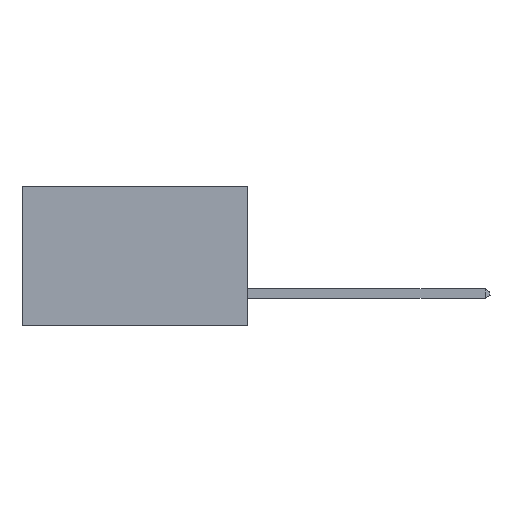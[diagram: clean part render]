
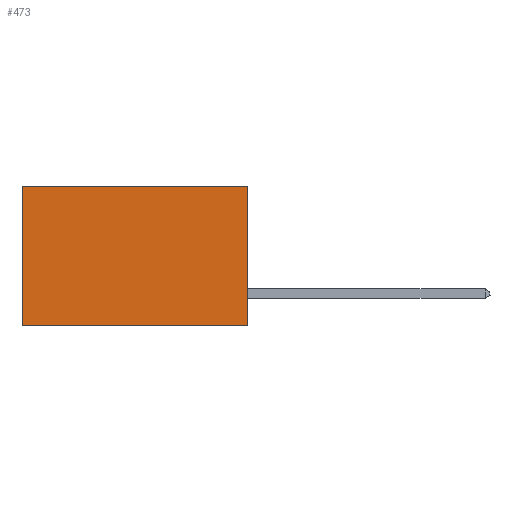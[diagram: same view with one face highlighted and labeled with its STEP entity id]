
A CAD part, left-side view. The second image highlights one B-rep face of the part: STEP entity #473.
In plain terms, the highlighted planar face has unit normal (-1, 0, 0).
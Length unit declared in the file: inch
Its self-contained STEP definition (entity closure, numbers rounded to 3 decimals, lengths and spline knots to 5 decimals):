
#473 = ADVANCED_FACE ( 'NONE', ( #12881 ), #9244, .F. ) ;
#481 = CARTESIAN_POINT ( 'NONE',  ( 0.298, 0., 0. ) ) ;
#1046 = DIRECTION ( 'NONE',  ( 0., 0., -1. ) ) ;
#2513 = VERTEX_POINT ( 'NONE', #10238 ) ;
#3491 = VECTOR ( 'NONE', #10605, 39.37008 ) ;
#3504 = LINE ( 'NONE', #19838, #8484 ) ;
#3913 = EDGE_LOOP ( 'NONE', ( #11380, #5056, #8881, #12155 ) ) ;
#5056 = ORIENTED_EDGE ( 'NONE', *, *, #7314, .F. ) ;
#5785 = CARTESIAN_POINT ( 'NONE',  ( 0.298, 0., -0.37 ) ) ;
#5967 = DIRECTION ( 'NONE',  ( 1., 0., 0. ) ) ;
#6348 = LINE ( 'NONE', #14496, #15275 ) ;
#6452 = CARTESIAN_POINT ( 'NONE',  ( 0.298, 0.6, -0.37 ) ) ;
#7308 = VERTEX_POINT ( 'NONE', #6452 ) ;
#7314 = EDGE_CURVE ( 'NONE', #9567, #7308, #3504, .T. ) ;
#8022 = DIRECTION ( 'NONE',  ( 0., 1., 0. ) ) ;
#8484 = VECTOR ( 'NONE', #8022, 39.37008 ) ;
#8881 = ORIENTED_EDGE ( 'NONE', *, *, #15723, .F. ) ;
#9244 = PLANE ( 'NONE',  #19241 ) ;
#9567 = VERTEX_POINT ( 'NONE', #5785 ) ;
#10238 = CARTESIAN_POINT ( 'NONE',  ( 0.298, 0.6, 0. ) ) ;
#10605 = DIRECTION ( 'NONE',  ( 0., 1., 0. ) ) ;
#10952 = CARTESIAN_POINT ( 'NONE',  ( 0.298, 0., 0. ) ) ;
#11116 = LINE ( 'NONE', #21141, #19218 ) ;
#11380 = ORIENTED_EDGE ( 'NONE', *, *, #20919, .T. ) ;
#12155 = ORIENTED_EDGE ( 'NONE', *, *, #16074, .T. ) ;
#12824 = DIRECTION ( 'NONE',  ( 0., 0., -1. ) ) ;
#12881 = FACE_OUTER_BOUND ( 'NONE', #3913, .T. ) ;
#14051 = VERTEX_POINT ( 'NONE', #21353 ) ;
#14496 = CARTESIAN_POINT ( 'NONE',  ( 0.298, 0.6, 0. ) ) ;
#15275 = VECTOR ( 'NONE', #12824, 39.37008 ) ;
#15723 = EDGE_CURVE ( 'NONE', #14051, #9567, #11116, .T. ) ;
#15801 = DIRECTION ( 'NONE',  ( 0., 0., -1. ) ) ;
#16074 = EDGE_CURVE ( 'NONE', #14051, #2513, #17364, .T. ) ;
#17364 = LINE ( 'NONE', #481, #3491 ) ;
#19218 = VECTOR ( 'NONE', #1046, 39.37008 ) ;
#19241 = AXIS2_PLACEMENT_3D ( 'NONE', #10952, #5967, #15801 ) ;
#19838 = CARTESIAN_POINT ( 'NONE',  ( 0.298, 0., -0.37 ) ) ;
#20919 = EDGE_CURVE ( 'NONE', #2513, #7308, #6348, .T. ) ;
#21141 = CARTESIAN_POINT ( 'NONE',  ( 0.298, 0., 0. ) ) ;
#21353 = CARTESIAN_POINT ( 'NONE',  ( 0.298, 0., 0. ) ) ;
